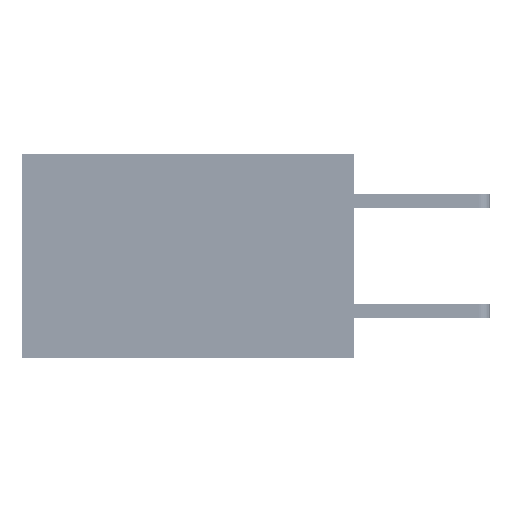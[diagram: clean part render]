
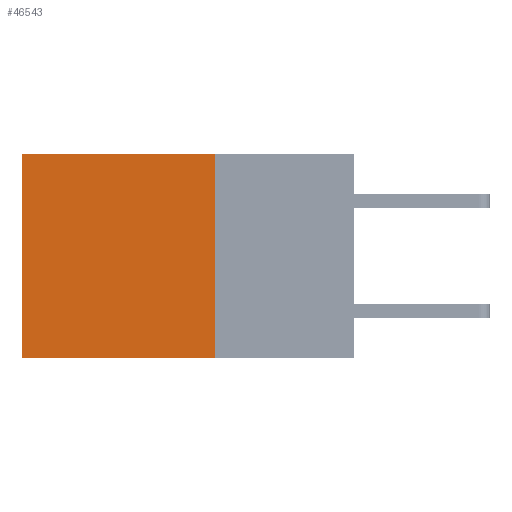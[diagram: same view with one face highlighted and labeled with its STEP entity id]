
A CAD part, left-side view. The second image highlights one B-rep face of the part: STEP entity #46543.
In plain terms, the highlighted planar face has unit normal (-1, 0, 0).
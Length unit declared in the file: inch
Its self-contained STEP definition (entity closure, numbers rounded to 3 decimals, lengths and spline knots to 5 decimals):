
#2609 = ORIENTED_EDGE ( 'NONE', *, *, #41299, .T. ) ;
#2919 = VERTEX_POINT ( 'NONE', #21602 ) ;
#4006 = FACE_OUTER_BOUND ( 'NONE', #16296, .T. ) ;
#5069 = VECTOR ( 'NONE', #14318, 39.37008 ) ;
#6522 = EDGE_CURVE ( 'NONE', #26468, #2919, #49949, .T. ) ;
#7319 = DIRECTION ( 'NONE',  ( 0., 1., 0. ) ) ;
#7546 = AXIS2_PLACEMENT_3D ( 'NONE', #49683, #32967, #41494 ) ;
#7656 = VERTEX_POINT ( 'NONE', #9319 ) ;
#8303 = CARTESIAN_POINT ( 'NONE',  ( 0.2875, 0.25, -0.37 ) ) ;
#9319 = CARTESIAN_POINT ( 'NONE',  ( 0.2875, 0.25, 0. ) ) ;
#10091 = ORIENTED_EDGE ( 'NONE', *, *, #44039, .F. ) ;
#14318 = DIRECTION ( 'NONE',  ( 0., 0., -1. ) ) ;
#14494 = CARTESIAN_POINT ( 'NONE',  ( 0.2875, 0.6, 0. ) ) ;
#15342 = VECTOR ( 'NONE', #28418, 39.37008 ) ;
#16296 = EDGE_LOOP ( 'NONE', ( #30360, #31346, #10091, #2609 ) ) ;
#17177 = PLANE ( 'NONE',  #7546 ) ;
#18343 = DIRECTION ( 'NONE',  ( 0., 0., -1. ) ) ;
#21329 = LINE ( 'NONE', #46464, #5069 ) ;
#21602 = CARTESIAN_POINT ( 'NONE',  ( 0.2875, 0.6, -0.37 ) ) ;
#23042 = VECTOR ( 'NONE', #18343, 39.37008 ) ;
#26468 = VERTEX_POINT ( 'NONE', #37284 ) ;
#28418 = DIRECTION ( 'NONE',  ( 0., 1., 0. ) ) ;
#30360 = ORIENTED_EDGE ( 'NONE', *, *, #6522, .T. ) ;
#31346 = ORIENTED_EDGE ( 'NONE', *, *, #32518, .F. ) ;
#32518 = EDGE_CURVE ( 'NONE', #42900, #2919, #50980, .T. ) ;
#32967 = DIRECTION ( 'NONE',  ( 1., 0., 0. ) ) ;
#37284 = CARTESIAN_POINT ( 'NONE',  ( 0.2875, 0.6, 0. ) ) ;
#39087 = VECTOR ( 'NONE', #7319, 39.37008 ) ;
#39354 = CARTESIAN_POINT ( 'NONE',  ( 0.2875, 0.25, 0. ) ) ;
#41299 = EDGE_CURVE ( 'NONE', #7656, #26468, #49696, .T. ) ;
#41494 = DIRECTION ( 'NONE',  ( 0., 0., -1. ) ) ;
#42900 = VERTEX_POINT ( 'NONE', #45424 ) ;
#44039 = EDGE_CURVE ( 'NONE', #7656, #42900, #21329, .T. ) ;
#45424 = CARTESIAN_POINT ( 'NONE',  ( 0.2875, 0.25, -0.37 ) ) ;
#46464 = CARTESIAN_POINT ( 'NONE',  ( 0.2875, 0.25, 0. ) ) ;
#46543 = ADVANCED_FACE ( 'NONE', ( #4006 ), #17177, .F. ) ;
#49683 = CARTESIAN_POINT ( 'NONE',  ( 0.2875, 0.25, 0. ) ) ;
#49696 = LINE ( 'NONE', #39354, #39087 ) ;
#49949 = LINE ( 'NONE', #14494, #23042 ) ;
#50980 = LINE ( 'NONE', #8303, #15342 ) ;
